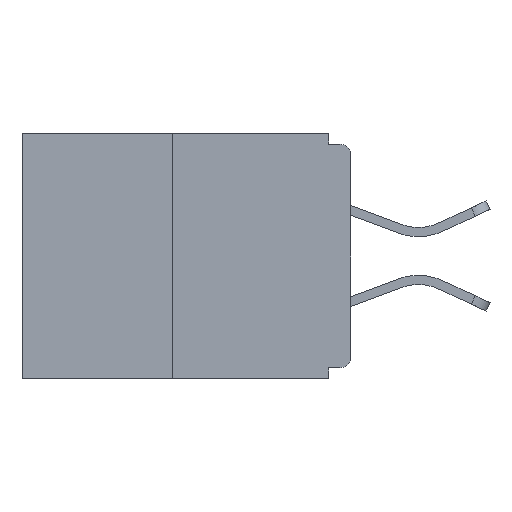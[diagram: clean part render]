
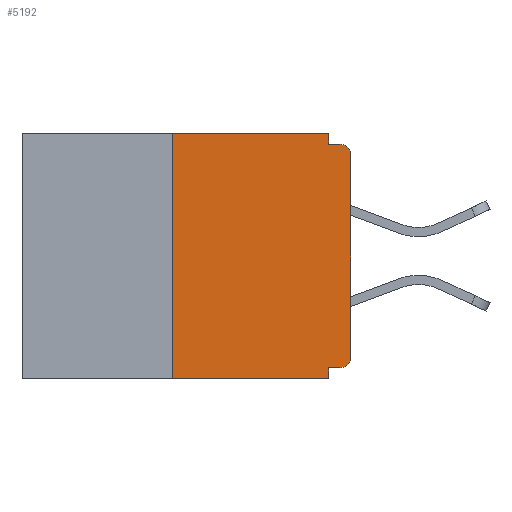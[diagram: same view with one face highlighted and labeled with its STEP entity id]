
A CAD part, left-side view. The second image highlights one B-rep face of the part: STEP entity #5192.
In plain terms, the highlighted planar face has unit normal (-1, 0, 0).
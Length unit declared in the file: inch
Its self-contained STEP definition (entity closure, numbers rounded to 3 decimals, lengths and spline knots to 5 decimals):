
#12 = VERTEX_POINT ( 'NONE', #20677 ) ;
#304 = DIRECTION ( 'NONE',  ( 0., -1., 0. ) ) ;
#1285 = VECTOR ( 'NONE', #5837, 39.37008 ) ;
#1347 = VERTEX_POINT ( 'NONE', #6958 ) ;
#1841 = CARTESIAN_POINT ( 'NONE',  ( 0., 0.031, -0.328 ) ) ;
#2371 = VERTEX_POINT ( 'NONE', #12251 ) ;
#2487 = CARTESIAN_POINT ( 'NONE',  ( 0., 0.46, -0.343 ) ) ;
#3457 = LINE ( 'NONE', #12353, #13481 ) ;
#4826 = EDGE_LOOP ( 'NONE', ( #26579, #8694, #27768, #5094, #19341, #11465, #11495, #7020, #22644, #8955 ) ) ;
#5089 = DIRECTION ( 'NONE',  ( 0., 0., -1. ) ) ;
#5094 = ORIENTED_EDGE ( 'NONE', *, *, #8424, .F. ) ;
#5192 = ADVANCED_FACE ( 'NONE', ( #21234 ), #16867, .F. ) ;
#5304 = VECTOR ( 'NONE', #26734, 39.37008 ) ;
#5837 = DIRECTION ( 'NONE',  ( 0., 0., -1. ) ) ;
#6212 = VERTEX_POINT ( 'NONE', #17652 ) ;
#6335 = LINE ( 'NONE', #25887, #10962 ) ;
#6412 = EDGE_CURVE ( 'NONE', #23240, #6212, #22448, .T. ) ;
#6896 = CARTESIAN_POINT ( 'NONE',  ( 0., 0.25, -0.343 ) ) ;
#6905 = DIRECTION ( 'NONE',  ( 0., -1., 0. ) ) ;
#6958 = CARTESIAN_POINT ( 'NONE',  ( 0., 0.25, 0. ) ) ;
#7020 = ORIENTED_EDGE ( 'NONE', *, *, #25628, .T. ) ;
#7127 = DIRECTION ( 'NONE',  ( 0., -1., 0. ) ) ;
#7278 = DIRECTION ( 'NONE',  ( -1., 0., 0. ) ) ;
#7336 = VERTEX_POINT ( 'NONE', #19945 ) ;
#7577 = VECTOR ( 'NONE', #11457, 39.37008 ) ;
#7909 = EDGE_CURVE ( 'NONE', #7336, #12878, #27072, .T. ) ;
#8424 = EDGE_CURVE ( 'NONE', #20552, #2371, #28827, .T. ) ;
#8694 = ORIENTED_EDGE ( 'NONE', *, *, #27222, .F. ) ;
#8925 = CARTESIAN_POINT ( 'NONE',  ( 0., 0.031, -0.343 ) ) ;
#8955 = ORIENTED_EDGE ( 'NONE', *, *, #21364, .F. ) ;
#9110 = VECTOR ( 'NONE', #6905, 39.37008 ) ;
#10004 = DIRECTION ( 'NONE',  ( 0., 0., -1. ) ) ;
#10033 = DIRECTION ( 'NONE',  ( 0., 0., 1. ) ) ;
#10060 = DIRECTION ( 'NONE',  ( -1., 0., 0. ) ) ;
#10576 = DIRECTION ( 'NONE',  ( 0., 1., 0. ) ) ;
#10579 = EDGE_CURVE ( 'NONE', #14486, #2371, #22189, .T. ) ;
#10962 = VECTOR ( 'NONE', #10576, 39.37008 ) ;
#11457 = DIRECTION ( 'NONE',  ( 0., 0., 1. ) ) ;
#11465 = ORIENTED_EDGE ( 'NONE', *, *, #15898, .T. ) ;
#11495 = ORIENTED_EDGE ( 'NONE', *, *, #7909, .T. ) ;
#12050 = CIRCLE ( 'NONE', #19053, 0.015 ) ;
#12251 = CARTESIAN_POINT ( 'NONE',  ( 0., 0.031, -0.343 ) ) ;
#12308 = CARTESIAN_POINT ( 'NONE',  ( 0., 0.015, -0.328 ) ) ;
#12353 = CARTESIAN_POINT ( 'NONE',  ( 0., 0.25, 0. ) ) ;
#12878 = VERTEX_POINT ( 'NONE', #13142 ) ;
#13142 = CARTESIAN_POINT ( 'NONE',  ( 0., 0., -0.03 ) ) ;
#13481 = VECTOR ( 'NONE', #10033, 39.37008 ) ;
#14486 = VERTEX_POINT ( 'NONE', #6896 ) ;
#14678 = CARTESIAN_POINT ( 'NONE',  ( 0., 0.46, 0. ) ) ;
#14721 = CARTESIAN_POINT ( 'NONE',  ( 0., 0.031, -0.015 ) ) ;
#15898 = EDGE_CURVE ( 'NONE', #17243, #7336, #21684, .T. ) ;
#16528 = EDGE_CURVE ( 'NONE', #17243, #20552, #6335, .T. ) ;
#16867 = PLANE ( 'NONE',  #22033 ) ;
#16948 = VECTOR ( 'NONE', #304, 39.37008 ) ;
#17243 = VERTEX_POINT ( 'NONE', #12308 ) ;
#17652 = CARTESIAN_POINT ( 'NONE',  ( 0., 0.015, -0.015 ) ) ;
#18739 = CARTESIAN_POINT ( 'NONE',  ( 0., 0., -0.015 ) ) ;
#18943 = DIRECTION ( 'NONE',  ( 0., 0., -1. ) ) ;
#19053 = AXIS2_PLACEMENT_3D ( 'NONE', #21142, #10060, #18943 ) ;
#19341 = ORIENTED_EDGE ( 'NONE', *, *, #16528, .F. ) ;
#19404 = CARTESIAN_POINT ( 'NONE',  ( 0., 0.031, 0. ) ) ;
#19945 = CARTESIAN_POINT ( 'NONE',  ( 0., 0., -0.313 ) ) ;
#20552 = VERTEX_POINT ( 'NONE', #1841 ) ;
#20677 = CARTESIAN_POINT ( 'NONE',  ( 0., 0.031, 0. ) ) ;
#21142 = CARTESIAN_POINT ( 'NONE',  ( 0., 0.015, -0.03 ) ) ;
#21234 = FACE_OUTER_BOUND ( 'NONE', #4826, .T. ) ;
#21364 = EDGE_CURVE ( 'NONE', #12, #23240, #25827, .T. ) ;
#21684 = CIRCLE ( 'NONE', #22130, 0.015 ) ;
#22033 = AXIS2_PLACEMENT_3D ( 'NONE', #14678, #25891, #10004 ) ;
#22045 = EDGE_CURVE ( 'NONE', #1347, #12, #26758, .T. ) ;
#22130 = AXIS2_PLACEMENT_3D ( 'NONE', #24953, #7278, #5089 ) ;
#22189 = LINE ( 'NONE', #2487, #24917 ) ;
#22448 = LINE ( 'NONE', #18739, #16948 ) ;
#22644 = ORIENTED_EDGE ( 'NONE', *, *, #6412, .F. ) ;
#22693 = CARTESIAN_POINT ( 'NONE',  ( 0., 0., 0. ) ) ;
#23240 = VERTEX_POINT ( 'NONE', #14721 ) ;
#24917 = VECTOR ( 'NONE', #7127, 39.37008 ) ;
#24953 = CARTESIAN_POINT ( 'NONE',  ( 0., 0.015, -0.313 ) ) ;
#25628 = EDGE_CURVE ( 'NONE', #12878, #6212, #12050, .T. ) ;
#25827 = LINE ( 'NONE', #19404, #1285 ) ;
#25887 = CARTESIAN_POINT ( 'NONE',  ( 0., 0., -0.328 ) ) ;
#25891 = DIRECTION ( 'NONE',  ( 1., 0., 0. ) ) ;
#26579 = ORIENTED_EDGE ( 'NONE', *, *, #22045, .F. ) ;
#26734 = DIRECTION ( 'NONE',  ( 0., 0., -1. ) ) ;
#26758 = LINE ( 'NONE', #26910, #9110 ) ;
#26910 = CARTESIAN_POINT ( 'NONE',  ( 0., 0.46, 0. ) ) ;
#27072 = LINE ( 'NONE', #22693, #7577 ) ;
#27222 = EDGE_CURVE ( 'NONE', #14486, #1347, #3457, .T. ) ;
#27768 = ORIENTED_EDGE ( 'NONE', *, *, #10579, .T. ) ;
#28827 = LINE ( 'NONE', #8925, #5304 ) ;
